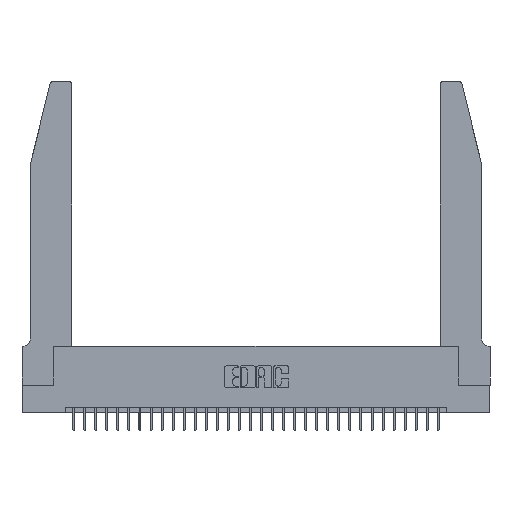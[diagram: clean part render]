
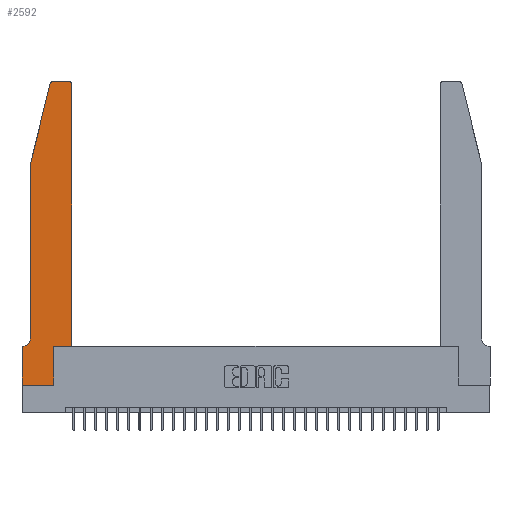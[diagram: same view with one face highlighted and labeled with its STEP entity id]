
A CAD part, top view. The second image highlights one B-rep face of the part: STEP entity #2592.
In plain terms, the highlighted planar face has unit normal (0, 0, 1).
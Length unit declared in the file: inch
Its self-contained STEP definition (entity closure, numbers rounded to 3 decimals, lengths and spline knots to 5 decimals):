
#138 = VERTEX_POINT ( 'NONE', #2051 ) ;
#146 = CARTESIAN_POINT ( 'NONE',  ( 0.2865, 0., 0.37 ) ) ;
#296 = CARTESIAN_POINT ( 'NONE',  ( 0.4205, 2.72, 0.37 ) ) ;
#327 = VERTEX_POINT ( 'NONE', #146 ) ;
#390 = EDGE_CURVE ( 'NONE', #30009, #20620, #18386, .T. ) ;
#1014 = CARTESIAN_POINT ( 'NONE',  ( 0.0755, 0.42, 0.37 ) ) ;
#1346 = CARTESIAN_POINT ( 'NONE',  ( 0., 0.35, 0.37 ) ) ;
#1666 = CARTESIAN_POINT ( 'NONE',  ( 0.4505, 0.35, 0.37 ) ) ;
#1753 = EDGE_CURVE ( 'NONE', #20620, #9780, #10059, .T. ) ;
#1997 = CARTESIAN_POINT ( 'NONE',  ( 0.0755, 2., 0.37 ) ) ;
#2051 = CARTESIAN_POINT ( 'NONE',  ( 0.4205, 2.75, 0.37 ) ) ;
#2386 = AXIS2_PLACEMENT_3D ( 'NONE', #296, #7805, #12877 ) ;
#2427 = CARTESIAN_POINT ( 'NONE',  ( 0.0055, 0.35, 0.37 ) ) ;
#2477 = DIRECTION ( 'NONE',  ( -1., 0., 0. ) ) ;
#2592 = ADVANCED_FACE ( 'NONE', ( #17862 ), #13789, .T. ) ;
#3011 = CARTESIAN_POINT ( 'NONE',  ( 0.0755, 2., 0.37 ) ) ;
#3203 = EDGE_CURVE ( 'NONE', #138, #13788, #11535, .T. ) ;
#3813 = DIRECTION ( 'NONE',  ( 0., 0., 1. ) ) ;
#4954 = VECTOR ( 'NONE', #26109, 39.37008 ) ;
#5050 = VERTEX_POINT ( 'NONE', #13275 ) ;
#5053 = DIRECTION ( 'NONE',  ( -1., 0., 0. ) ) ;
#5188 = AXIS2_PLACEMENT_3D ( 'NONE', #17648, #30325, #20723 ) ;
#5892 = VECTOR ( 'NONE', #2477, 39.37008 ) ;
#6012 = ORIENTED_EDGE ( 'NONE', *, *, #10042, .T. ) ;
#6482 = DIRECTION ( 'NONE',  ( 0., 1., 0. ) ) ;
#6815 = LINE ( 'NONE', #26467, #5892 ) ;
#7374 = LINE ( 'NONE', #18988, #10148 ) ;
#7805 = DIRECTION ( 'NONE',  ( 0., 0., 1. ) ) ;
#8362 = ORIENTED_EDGE ( 'NONE', *, *, #3203, .T. ) ;
#8656 = VERTEX_POINT ( 'NONE', #1997 ) ;
#8686 = EDGE_CURVE ( 'NONE', #5050, #8656, #27335, .T. ) ;
#9365 = EDGE_CURVE ( 'NONE', #31441, #327, #28465, .T. ) ;
#9635 = VERTEX_POINT ( 'NONE', #1014 ) ;
#9777 = VECTOR ( 'NONE', #31296, 39.37008 ) ;
#9780 = VERTEX_POINT ( 'NONE', #28964 ) ;
#10042 = EDGE_CURVE ( 'NONE', #9635, #27282, #31322, .T. ) ;
#10048 = EDGE_CURVE ( 'NONE', #13788, #5050, #20267, .T. ) ;
#10059 = LINE ( 'NONE', #28439, #4954 ) ;
#10148 = VECTOR ( 'NONE', #6482, 39.37008 ) ;
#10221 = CARTESIAN_POINT ( 'NONE',  ( 0.0755, 2., 0.37 ) ) ;
#10408 = AXIS2_PLACEMENT_3D ( 'NONE', #1346, #3813, #21348 ) ;
#10715 = CARTESIAN_POINT ( 'NONE',  ( 0., 0., 0.37 ) ) ;
#10802 = DIRECTION ( 'NONE',  ( 0., 0., 1. ) ) ;
#11085 = CARTESIAN_POINT ( 'NONE',  ( 0., 0., 0.37 ) ) ;
#11535 = LINE ( 'NONE', #22507, #22840 ) ;
#12397 = ORIENTED_EDGE ( 'NONE', *, *, #8686, .T. ) ;
#12877 = DIRECTION ( 'NONE',  ( 1., 0., 0. ) ) ;
#13275 = CARTESIAN_POINT ( 'NONE',  ( 0.25487, 2.72718, 0.37 ) ) ;
#13297 = DIRECTION ( 'NONE',  ( 0., -1., 0. ) ) ;
#13547 = CARTESIAN_POINT ( 'NONE',  ( 0., 0.35, 0.37 ) ) ;
#13636 = ORIENTED_EDGE ( 'NONE', *, *, #21967, .T. ) ;
#13697 = CARTESIAN_POINT ( 'NONE',  ( 0.4505, 0.35, 0.37 ) ) ;
#13788 = VERTEX_POINT ( 'NONE', #25316 ) ;
#13789 = PLANE ( 'NONE',  #10408 ) ;
#13829 = EDGE_CURVE ( 'NONE', #327, #30009, #7374, .T. ) ;
#15235 = DIRECTION ( 'NONE',  ( 0., -1., 0. ) ) ;
#15936 = ORIENTED_EDGE ( 'NONE', *, *, #18515, .T. ) ;
#15982 = DIRECTION ( 'NONE',  ( 1., 0., 0. ) ) ;
#16772 = EDGE_LOOP ( 'NONE', ( #8362, #25900, #12397, #29473, #6012, #31453, #13636, #27308, #25360, #31352, #26533, #15936 ) ) ;
#16825 = VECTOR ( 'NONE', #15235, 39.37008 ) ;
#17536 = CARTESIAN_POINT ( 'NONE',  ( 0.2865, 0.35, 0.37 ) ) ;
#17648 = CARTESIAN_POINT ( 'NONE',  ( 0.0055, 0.42, 0.37 ) ) ;
#17785 = DIRECTION ( 'NONE',  ( -0.239, -0.971, 0. ) ) ;
#17862 = FACE_OUTER_BOUND ( 'NONE', #16772, .T. ) ;
#18386 = LINE ( 'NONE', #13697, #9777 ) ;
#18515 = EDGE_CURVE ( 'NONE', #9780, #138, #28317, .T. ) ;
#18649 = AXIS2_PLACEMENT_3D ( 'NONE', #20137, #10802, #25114 ) ;
#18988 = CARTESIAN_POINT ( 'NONE',  ( 0.2865, 0.35, 0.37 ) ) ;
#20137 = CARTESIAN_POINT ( 'NONE',  ( 0.284, 2.72, 0.37 ) ) ;
#20267 = CIRCLE ( 'NONE', #18649, 0.03 ) ;
#20602 = VECTOR ( 'NONE', #17785, 39.37008 ) ;
#20620 = VERTEX_POINT ( 'NONE', #1666 ) ;
#20723 = DIRECTION ( 'NONE',  ( -1., 0., 0. ) ) ;
#21348 = DIRECTION ( 'NONE',  ( 1., 0., 0. ) ) ;
#21967 = EDGE_CURVE ( 'NONE', #26069, #31441, #24154, .T. ) ;
#22507 = CARTESIAN_POINT ( 'NONE',  ( 0.2605, 2.75, 0.37 ) ) ;
#22840 = VECTOR ( 'NONE', #5053, 39.37008 ) ;
#23686 = VECTOR ( 'NONE', #15982, 39.37008 ) ;
#24154 = LINE ( 'NONE', #11085, #29304 ) ;
#25114 = DIRECTION ( 'NONE',  ( 1., 0., 0. ) ) ;
#25316 = CARTESIAN_POINT ( 'NONE',  ( 0.284, 2.75, 0.37 ) ) ;
#25360 = ORIENTED_EDGE ( 'NONE', *, *, #13829, .T. ) ;
#25900 = ORIENTED_EDGE ( 'NONE', *, *, #10048, .T. ) ;
#26048 = CARTESIAN_POINT ( 'NONE',  ( 0., 0., 0.37 ) ) ;
#26069 = VERTEX_POINT ( 'NONE', #13547 ) ;
#26109 = DIRECTION ( 'NONE',  ( 0., 1., 0. ) ) ;
#26467 = CARTESIAN_POINT ( 'NONE',  ( 0.0755, 0.35, 0.37 ) ) ;
#26533 = ORIENTED_EDGE ( 'NONE', *, *, #1753, .T. ) ;
#27282 = VERTEX_POINT ( 'NONE', #2427 ) ;
#27308 = ORIENTED_EDGE ( 'NONE', *, *, #9365, .T. ) ;
#27335 = LINE ( 'NONE', #10221, #20602 ) ;
#28317 = CIRCLE ( 'NONE', #2386, 0.03 ) ;
#28439 = CARTESIAN_POINT ( 'NONE',  ( 0.4505, 0.35, 0.37 ) ) ;
#28465 = LINE ( 'NONE', #10715, #23686 ) ;
#28964 = CARTESIAN_POINT ( 'NONE',  ( 0.4505, 2.72, 0.37 ) ) ;
#29304 = VECTOR ( 'NONE', #13297, 39.37008 ) ;
#29473 = ORIENTED_EDGE ( 'NONE', *, *, #32024, .T. ) ;
#30009 = VERTEX_POINT ( 'NONE', #17536 ) ;
#30066 = EDGE_CURVE ( 'NONE', #27282, #26069, #6815, .T. ) ;
#30325 = DIRECTION ( 'NONE',  ( 0., 0., -1. ) ) ;
#31000 = LINE ( 'NONE', #3011, #16825 ) ;
#31296 = DIRECTION ( 'NONE',  ( 1., 0., 0. ) ) ;
#31322 = CIRCLE ( 'NONE', #5188, 0.07 ) ;
#31352 = ORIENTED_EDGE ( 'NONE', *, *, #390, .T. ) ;
#31441 = VERTEX_POINT ( 'NONE', #26048 ) ;
#31453 = ORIENTED_EDGE ( 'NONE', *, *, #30066, .T. ) ;
#32024 = EDGE_CURVE ( 'NONE', #8656, #9635, #31000, .T. ) ;
